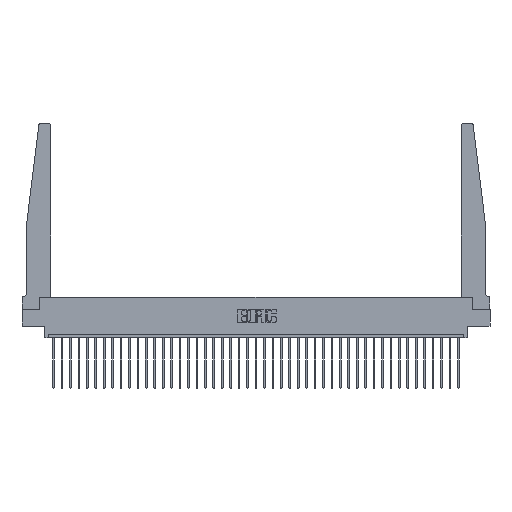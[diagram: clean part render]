
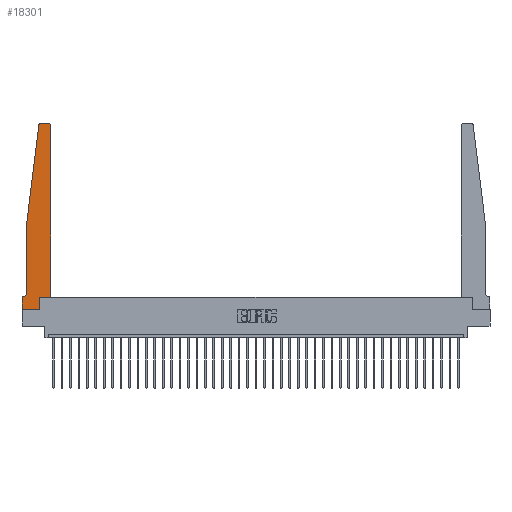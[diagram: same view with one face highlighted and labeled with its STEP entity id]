
A CAD part, top view. The second image highlights one B-rep face of the part: STEP entity #18301.
In plain terms, the highlighted planar face has unit normal (0, 0, 1).
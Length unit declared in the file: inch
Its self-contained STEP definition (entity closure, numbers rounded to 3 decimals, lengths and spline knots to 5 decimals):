
#528 = DIRECTION ( 'NONE',  ( -1., 0., 0. ) ) ;
#745 = EDGE_CURVE ( 'NONE', #33931, #13256, #9967, .T. ) ;
#794 = VERTEX_POINT ( 'NONE', #30050 ) ;
#1020 = DIRECTION ( 'NONE',  ( -0.122, -0.992, 0. ) ) ;
#1129 = CARTESIAN_POINT ( 'NONE',  ( 0., 0., 0.37 ) ) ;
#1193 = VERTEX_POINT ( 'NONE', #15518 ) ;
#1235 = EDGE_CURVE ( 'NONE', #17304, #26974, #6036, .T. ) ;
#1249 = ORIENTED_EDGE ( 'NONE', *, *, #7919, .T. ) ;
#1848 = EDGE_CURVE ( 'NONE', #3688, #33076, #12267, .T. ) ;
#2136 = LINE ( 'NONE', #12885, #13129 ) ;
#2404 = VECTOR ( 'NONE', #30422, 39.37008 ) ;
#3609 = ORIENTED_EDGE ( 'NONE', *, *, #17077, .T. ) ;
#3649 = VECTOR ( 'NONE', #23325, 39.37008 ) ;
#3688 = VERTEX_POINT ( 'NONE', #8356 ) ;
#3826 = EDGE_CURVE ( 'NONE', #19272, #13701, #19050, .T. ) ;
#4066 = CARTESIAN_POINT ( 'NONE',  ( 0.27653, 2.75, 0.37 ) ) ;
#4598 = PLANE ( 'NONE',  #13296 ) ;
#4637 = AXIS2_PLACEMENT_3D ( 'NONE', #20537, #12313, #9678 ) ;
#4911 = AXIS2_PLACEMENT_3D ( 'NONE', #5689, #5859, #32480 ) ;
#5471 = LINE ( 'NONE', #16165, #25435 ) ;
#5689 = CARTESIAN_POINT ( 'NONE',  ( 0.395, 2.72, 0.37 ) ) ;
#5755 = CARTESIAN_POINT ( 'NONE',  ( 0.065, 0.1875, 0.37 ) ) ;
#5859 = DIRECTION ( 'NONE',  ( 0., 0., 1. ) ) ;
#6036 = CIRCLE ( 'NONE', #4911, 0.03 ) ;
#6149 = CARTESIAN_POINT ( 'NONE',  ( 0., 0.1875, 0.37 ) ) ;
#7761 = DIRECTION ( 'NONE',  ( 1., 0., 0. ) ) ;
#7919 = EDGE_CURVE ( 'NONE', #14131, #3688, #30515, .T. ) ;
#8356 = CARTESIAN_POINT ( 'NONE',  ( 0.24675, 2.72367, 0.37 ) ) ;
#8410 = LINE ( 'NONE', #5755, #2404 ) ;
#8814 = ORIENTED_EDGE ( 'NONE', *, *, #745, .T. ) ;
#9455 = ORIENTED_EDGE ( 'NONE', *, *, #19261, .T. ) ;
#9646 = ORIENTED_EDGE ( 'NONE', *, *, #19169, .T. ) ;
#9678 = DIRECTION ( 'NONE',  ( 1., 0., 0. ) ) ;
#9967 = LINE ( 'NONE', #26327, #20029 ) ;
#9986 = EDGE_CURVE ( 'NONE', #27026, #19272, #8410, .T. ) ;
#10419 = VECTOR ( 'NONE', #15109, 39.37008 ) ;
#11162 = VECTOR ( 'NONE', #22058, 39.37008 ) ;
#12267 = LINE ( 'NONE', #19996, #25187 ) ;
#12313 = DIRECTION ( 'NONE',  ( 0., 0., 1. ) ) ;
#12775 = LINE ( 'NONE', #16066, #3649 ) ;
#12861 = LINE ( 'NONE', #28709, #10419 ) ;
#12885 = CARTESIAN_POINT ( 'NONE',  ( 0.425, 0.18, 0.37 ) ) ;
#13129 = VECTOR ( 'NONE', #34393, 39.37008 ) ;
#13256 = VERTEX_POINT ( 'NONE', #27443 ) ;
#13296 = AXIS2_PLACEMENT_3D ( 'NONE', #34377, #23764, #7761 ) ;
#13701 = VERTEX_POINT ( 'NONE', #1129 ) ;
#13717 = CARTESIAN_POINT ( 'NONE',  ( 0.015, 0.2375, 0.37 ) ) ;
#14044 = CARTESIAN_POINT ( 'NONE',  ( 0.425, 2.72, 0.37 ) ) ;
#14131 = VERTEX_POINT ( 'NONE', #4066 ) ;
#15109 = DIRECTION ( 'NONE',  ( -1., 0., 0. ) ) ;
#15518 = CARTESIAN_POINT ( 'NONE',  ( 0.065, 0.2375, 0.37 ) ) ;
#16066 = CARTESIAN_POINT ( 'NONE',  ( 0., 0., 0.37 ) ) ;
#16165 = CARTESIAN_POINT ( 'NONE',  ( 0.2605, 0.18, 0.37 ) ) ;
#16424 = EDGE_CURVE ( 'NONE', #13701, #794, #12775, .T. ) ;
#17077 = EDGE_CURVE ( 'NONE', #26974, #14131, #12861, .T. ) ;
#17304 = VERTEX_POINT ( 'NONE', #14044 ) ;
#18152 = CARTESIAN_POINT ( 'NONE',  ( 0.065, 1.25, 0.37 ) ) ;
#18301 = ADVANCED_FACE ( 'NONE', ( #26409 ), #4598, .T. ) ;
#18676 = CARTESIAN_POINT ( 'NONE',  ( 0.395, 2.75, 0.37 ) ) ;
#19050 = LINE ( 'NONE', #29848, #11162 ) ;
#19169 = EDGE_CURVE ( 'NONE', #33076, #1193, #26933, .T. ) ;
#19261 = EDGE_CURVE ( 'NONE', #1193, #27026, #25666, .T. ) ;
#19272 = VERTEX_POINT ( 'NONE', #6149 ) ;
#19528 = AXIS2_PLACEMENT_3D ( 'NONE', #13717, #21821, #528 ) ;
#19996 = CARTESIAN_POINT ( 'NONE',  ( 0.065, 1.25, 0.37 ) ) ;
#20029 = VECTOR ( 'NONE', #26494, 39.37008 ) ;
#20537 = CARTESIAN_POINT ( 'NONE',  ( 0.27653, 2.72, 0.37 ) ) ;
#20669 = ORIENTED_EDGE ( 'NONE', *, *, #31282, .T. ) ;
#20702 = ORIENTED_EDGE ( 'NONE', *, *, #9986, .T. ) ;
#21460 = ORIENTED_EDGE ( 'NONE', *, *, #16424, .T. ) ;
#21821 = DIRECTION ( 'NONE',  ( 0., 0., -1. ) ) ;
#22058 = DIRECTION ( 'NONE',  ( 0., -1., 0. ) ) ;
#23325 = DIRECTION ( 'NONE',  ( 1., 0., 0. ) ) ;
#23596 = DIRECTION ( 'NONE',  ( 0., -1., 0. ) ) ;
#23764 = DIRECTION ( 'NONE',  ( 0., 0., 1. ) ) ;
#24190 = CARTESIAN_POINT ( 'NONE',  ( 0.2605, 0.18, 0.37 ) ) ;
#24641 = DIRECTION ( 'NONE',  ( 0., 1., 0. ) ) ;
#25187 = VECTOR ( 'NONE', #1020, 39.37008 ) ;
#25435 = VECTOR ( 'NONE', #24641, 39.37008 ) ;
#25666 = CIRCLE ( 'NONE', #19528, 0.05 ) ;
#26273 = CARTESIAN_POINT ( 'NONE',  ( 0.015, 0.1875, 0.37 ) ) ;
#26327 = CARTESIAN_POINT ( 'NONE',  ( 0.425, 0.18, 0.37 ) ) ;
#26409 = FACE_OUTER_BOUND ( 'NONE', #30900, .T. ) ;
#26494 = DIRECTION ( 'NONE',  ( 1., 0., 0. ) ) ;
#26933 = LINE ( 'NONE', #31554, #29045 ) ;
#26974 = VERTEX_POINT ( 'NONE', #18676 ) ;
#27026 = VERTEX_POINT ( 'NONE', #26273 ) ;
#27443 = CARTESIAN_POINT ( 'NONE',  ( 0.425, 0.18, 0.37 ) ) ;
#28366 = ORIENTED_EDGE ( 'NONE', *, *, #1848, .T. ) ;
#28709 = CARTESIAN_POINT ( 'NONE',  ( 0.25, 2.75, 0.37 ) ) ;
#28755 = ORIENTED_EDGE ( 'NONE', *, *, #28910, .T. ) ;
#28910 = EDGE_CURVE ( 'NONE', #794, #33931, #5471, .T. ) ;
#29045 = VECTOR ( 'NONE', #23596, 39.37008 ) ;
#29848 = CARTESIAN_POINT ( 'NONE',  ( 0., 0., 0.37 ) ) ;
#30050 = CARTESIAN_POINT ( 'NONE',  ( 0.2605, 0., 0.37 ) ) ;
#30422 = DIRECTION ( 'NONE',  ( -1., 0., 0. ) ) ;
#30515 = CIRCLE ( 'NONE', #4637, 0.03 ) ;
#30900 = EDGE_LOOP ( 'NONE', ( #3609, #1249, #28366, #9646, #9455, #20702, #31410, #21460, #28755, #8814, #20669, #34086 ) ) ;
#31282 = EDGE_CURVE ( 'NONE', #13256, #17304, #2136, .T. ) ;
#31410 = ORIENTED_EDGE ( 'NONE', *, *, #3826, .T. ) ;
#31554 = CARTESIAN_POINT ( 'NONE',  ( 0.065, 1.25, 0.37 ) ) ;
#32480 = DIRECTION ( 'NONE',  ( 1., 0., 0. ) ) ;
#33076 = VERTEX_POINT ( 'NONE', #18152 ) ;
#33931 = VERTEX_POINT ( 'NONE', #24190 ) ;
#34086 = ORIENTED_EDGE ( 'NONE', *, *, #1235, .T. ) ;
#34377 = CARTESIAN_POINT ( 'NONE',  ( 0., 0.1875, 0.37 ) ) ;
#34393 = DIRECTION ( 'NONE',  ( 0., 1., 0. ) ) ;
